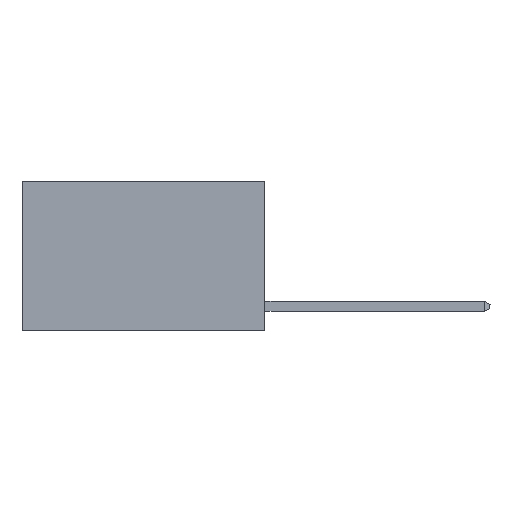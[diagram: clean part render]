
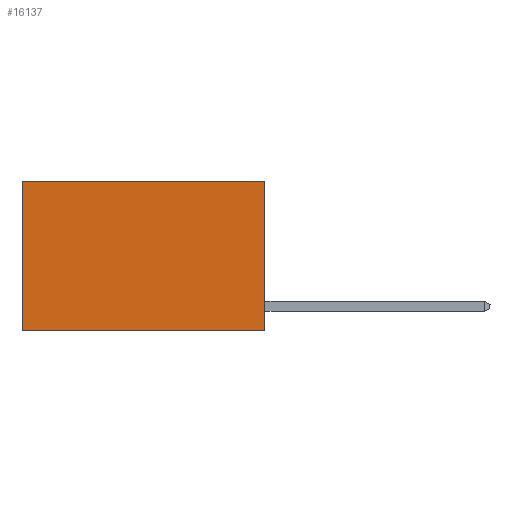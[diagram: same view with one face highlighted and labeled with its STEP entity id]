
A CAD part, left-side view. The second image highlights one B-rep face of the part: STEP entity #16137.
In plain terms, the highlighted planar face has unit normal (-1, 0, 0).
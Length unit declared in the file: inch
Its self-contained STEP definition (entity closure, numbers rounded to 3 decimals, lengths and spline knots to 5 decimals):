
#25 = VERTEX_POINT ( 'NONE', #18922 ) ;
#1258 = FACE_OUTER_BOUND ( 'NONE', #14058, .T. ) ;
#1785 = VECTOR ( 'NONE', #7431, 39.37008 ) ;
#3781 = DIRECTION ( 'NONE',  ( 0., 0., -1. ) ) ;
#4299 = VERTEX_POINT ( 'NONE', #11696 ) ;
#5112 = EDGE_CURVE ( 'NONE', #17808, #7179, #21304, .T. ) ;
#6850 = LINE ( 'NONE', #14743, #1785 ) ;
#7151 = LINE ( 'NONE', #9629, #21149 ) ;
#7179 = VERTEX_POINT ( 'NONE', #12643 ) ;
#7431 = DIRECTION ( 'NONE',  ( 0., 1., 0. ) ) ;
#8335 = EDGE_CURVE ( 'NONE', #7179, #4299, #7151, .T. ) ;
#9106 = CARTESIAN_POINT ( 'NONE',  ( 0.2625, 0., 0. ) ) ;
#9334 = AXIS2_PLACEMENT_3D ( 'NONE', #13078, #14892, #3781 ) ;
#9629 = CARTESIAN_POINT ( 'NONE',  ( 0.2625, 0.6, 0. ) ) ;
#10168 = EDGE_CURVE ( 'NONE', #25, #4299, #6850, .T. ) ;
#11250 = VECTOR ( 'NONE', #23452, 39.37008 ) ;
#11668 = VECTOR ( 'NONE', #20737, 39.37008 ) ;
#11696 = CARTESIAN_POINT ( 'NONE',  ( 0.2625, 0.6, -0.37 ) ) ;
#12643 = CARTESIAN_POINT ( 'NONE',  ( 0.2625, 0.6, 0. ) ) ;
#13078 = CARTESIAN_POINT ( 'NONE',  ( 0.2625, 0., 0. ) ) ;
#14058 = EDGE_LOOP ( 'NONE', ( #15706, #19154, #14431, #14655 ) ) ;
#14431 = ORIENTED_EDGE ( 'NONE', *, *, #17056, .F. ) ;
#14655 = ORIENTED_EDGE ( 'NONE', *, *, #5112, .T. ) ;
#14743 = CARTESIAN_POINT ( 'NONE',  ( 0.2625, 0., -0.37 ) ) ;
#14892 = DIRECTION ( 'NONE',  ( 1., 0., 0. ) ) ;
#15706 = ORIENTED_EDGE ( 'NONE', *, *, #8335, .T. ) ;
#16137 = ADVANCED_FACE ( 'NONE', ( #1258 ), #23860, .F. ) ;
#17056 = EDGE_CURVE ( 'NONE', #17808, #25, #21446, .T. ) ;
#17808 = VERTEX_POINT ( 'NONE', #9106 ) ;
#18922 = CARTESIAN_POINT ( 'NONE',  ( 0.2625, 0., -0.37 ) ) ;
#19154 = ORIENTED_EDGE ( 'NONE', *, *, #10168, .F. ) ;
#20532 = DIRECTION ( 'NONE',  ( 0., 0., -1. ) ) ;
#20737 = DIRECTION ( 'NONE',  ( 0., 1., 0. ) ) ;
#20816 = CARTESIAN_POINT ( 'NONE',  ( 0.2625, 0., 0. ) ) ;
#21149 = VECTOR ( 'NONE', #20532, 39.37008 ) ;
#21304 = LINE ( 'NONE', #20816, #11668 ) ;
#21446 = LINE ( 'NONE', #21683, #11250 ) ;
#21683 = CARTESIAN_POINT ( 'NONE',  ( 0.2625, 0., 0. ) ) ;
#23452 = DIRECTION ( 'NONE',  ( 0., 0., -1. ) ) ;
#23860 = PLANE ( 'NONE',  #9334 ) ;
